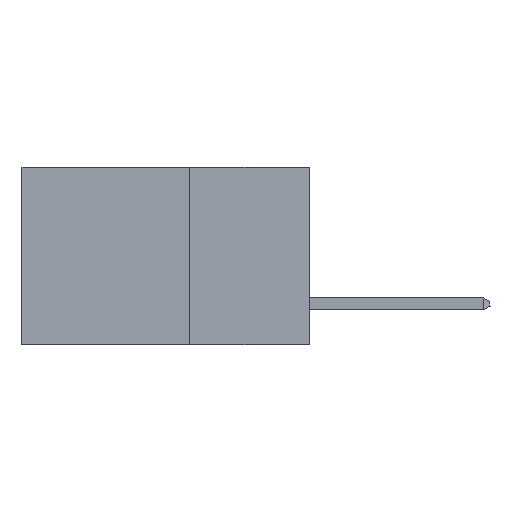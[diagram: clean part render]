
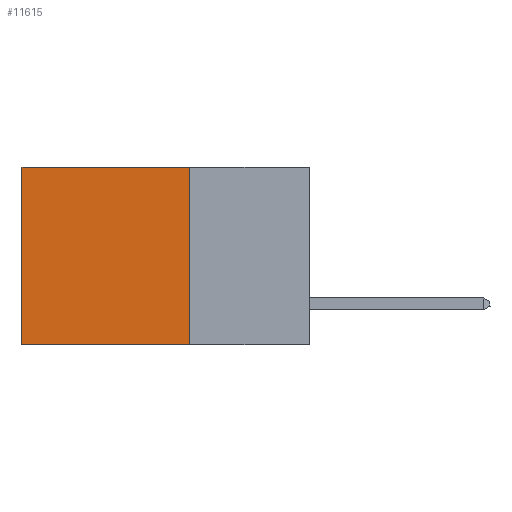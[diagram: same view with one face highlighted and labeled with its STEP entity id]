
A CAD part, left-side view. The second image highlights one B-rep face of the part: STEP entity #11615.
In plain terms, the highlighted planar face has unit normal (-1, 0, 0).
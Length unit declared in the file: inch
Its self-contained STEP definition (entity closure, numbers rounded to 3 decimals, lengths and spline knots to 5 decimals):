
#299 = ORIENTED_EDGE ( 'NONE', *, *, #6981, .T. ) ;
#727 = CARTESIAN_POINT ( 'NONE',  ( 0.2875, 0.25, -0.37 ) ) ;
#1186 = PLANE ( 'NONE',  #14114 ) ;
#2219 = DIRECTION ( 'NONE',  ( 0., 0., -1. ) ) ;
#2608 = VERTEX_POINT ( 'NONE', #8205 ) ;
#2618 = DIRECTION ( 'NONE',  ( 1., 0., 0. ) ) ;
#2847 = VECTOR ( 'NONE', #15262, 39.37008 ) ;
#4047 = VECTOR ( 'NONE', #6317, 39.37008 ) ;
#4087 = VERTEX_POINT ( 'NONE', #10365 ) ;
#4116 = CARTESIAN_POINT ( 'NONE',  ( 0.2875, 0.6, 0. ) ) ;
#4469 = LINE ( 'NONE', #727, #4047 ) ;
#5666 = CARTESIAN_POINT ( 'NONE',  ( 0.2875, 0.25, 0. ) ) ;
#6317 = DIRECTION ( 'NONE',  ( 0., 1., 0. ) ) ;
#6470 = VERTEX_POINT ( 'NONE', #17128 ) ;
#6981 = EDGE_CURVE ( 'NONE', #6470, #2608, #14872, .T. ) ;
#7055 = DIRECTION ( 'NONE',  ( 0., 1., 0. ) ) ;
#8205 = CARTESIAN_POINT ( 'NONE',  ( 0.2875, 0.6, 0. ) ) ;
#8576 = EDGE_CURVE ( 'NONE', #6470, #4087, #13732, .T. ) ;
#9169 = CARTESIAN_POINT ( 'NONE',  ( 0.2875, 0.25, 0. ) ) ;
#9503 = ORIENTED_EDGE ( 'NONE', *, *, #10402, .F. ) ;
#9988 = VECTOR ( 'NONE', #2219, 39.37008 ) ;
#10121 = FACE_OUTER_BOUND ( 'NONE', #14832, .T. ) ;
#10365 = CARTESIAN_POINT ( 'NONE',  ( 0.2875, 0.25, -0.37 ) ) ;
#10381 = ORIENTED_EDGE ( 'NONE', *, *, #8576, .F. ) ;
#10402 = EDGE_CURVE ( 'NONE', #4087, #13379, #4469, .T. ) ;
#10728 = LINE ( 'NONE', #4116, #2847 ) ;
#11005 = CARTESIAN_POINT ( 'NONE',  ( 0.2875, 0.25, 0. ) ) ;
#11615 = ADVANCED_FACE ( 'NONE', ( #10121 ), #1186, .F. ) ;
#12443 = DIRECTION ( 'NONE',  ( 0., 0., -1. ) ) ;
#13379 = VERTEX_POINT ( 'NONE', #13760 ) ;
#13732 = LINE ( 'NONE', #9169, #9988 ) ;
#13760 = CARTESIAN_POINT ( 'NONE',  ( 0.2875, 0.6, -0.37 ) ) ;
#14114 = AXIS2_PLACEMENT_3D ( 'NONE', #11005, #2618, #12443 ) ;
#14551 = ORIENTED_EDGE ( 'NONE', *, *, #16600, .T. ) ;
#14832 = EDGE_LOOP ( 'NONE', ( #14551, #9503, #10381, #299 ) ) ;
#14872 = LINE ( 'NONE', #5666, #15284 ) ;
#15262 = DIRECTION ( 'NONE',  ( 0., 0., -1. ) ) ;
#15284 = VECTOR ( 'NONE', #7055, 39.37008 ) ;
#16600 = EDGE_CURVE ( 'NONE', #2608, #13379, #10728, .T. ) ;
#17128 = CARTESIAN_POINT ( 'NONE',  ( 0.2875, 0.25, 0. ) ) ;
